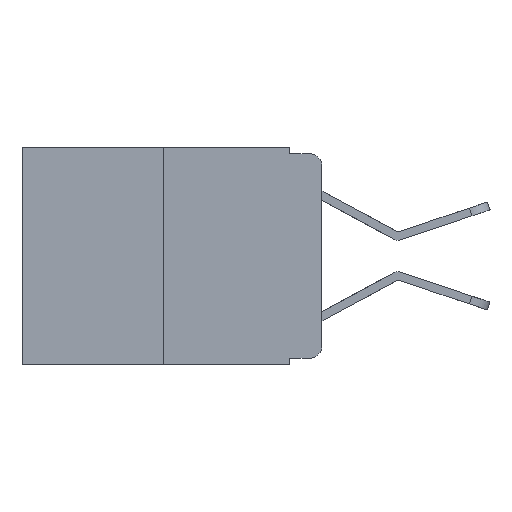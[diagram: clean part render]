
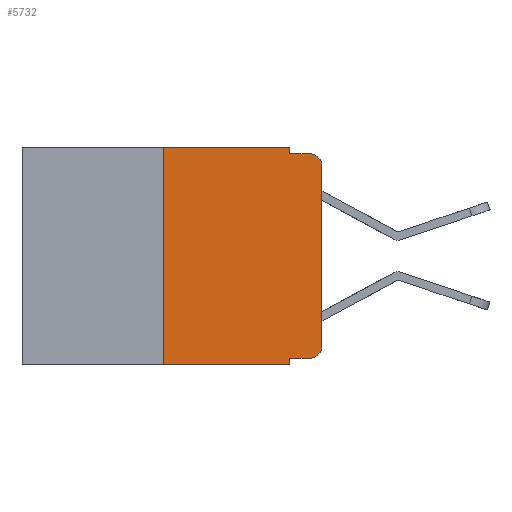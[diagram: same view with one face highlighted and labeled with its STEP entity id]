
A CAD part, left-side view. The second image highlights one B-rep face of the part: STEP entity #5732.
In plain terms, the highlighted planar face has unit normal (-1, 0, 0).
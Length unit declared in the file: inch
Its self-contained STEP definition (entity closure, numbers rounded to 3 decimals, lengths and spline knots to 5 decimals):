
#73 = LINE ( 'NONE', #10093, #9554 ) ;
#225 = VERTEX_POINT ( 'NONE', #10818 ) ;
#378 = EDGE_CURVE ( 'NONE', #3443, #225, #941, .T. ) ;
#417 = VECTOR ( 'NONE', #4463, 39.37008 ) ;
#472 = ORIENTED_EDGE ( 'NONE', *, *, #11811, .T. ) ;
#626 = VECTOR ( 'NONE', #1200, 39.37008 ) ;
#719 = CARTESIAN_POINT ( 'NONE',  ( 0., 0.051, -0.01 ) ) ;
#941 = LINE ( 'NONE', #6749, #626 ) ;
#1099 = VECTOR ( 'NONE', #4678, 39.37008 ) ;
#1198 = ORIENTED_EDGE ( 'NONE', *, *, #8436, .F. ) ;
#1200 = DIRECTION ( 'NONE',  ( 0., -1., 0. ) ) ;
#1203 = LINE ( 'NONE', #6163, #10564 ) ;
#1579 = VERTEX_POINT ( 'NONE', #11985 ) ;
#1754 = LINE ( 'NONE', #3778, #6861 ) ;
#1831 = AXIS2_PLACEMENT_3D ( 'NONE', #8529, #10321, #4838 ) ;
#1996 = VECTOR ( 'NONE', #5301, 39.37008 ) ;
#2070 = VERTEX_POINT ( 'NONE', #5599 ) ;
#2084 = EDGE_CURVE ( 'NONE', #9857, #3443, #4594, .T. ) ;
#2336 = AXIS2_PLACEMENT_3D ( 'NONE', #2449, #9038, #3432 ) ;
#2449 = CARTESIAN_POINT ( 'NONE',  ( 0., 0.02, -0.313 ) ) ;
#2727 = CARTESIAN_POINT ( 'NONE',  ( 0., 0.051, -0.01 ) ) ;
#2762 = ORIENTED_EDGE ( 'NONE', *, *, #378, .F. ) ;
#2826 = ORIENTED_EDGE ( 'NONE', *, *, #7855, .T. ) ;
#2958 = ORIENTED_EDGE ( 'NONE', *, *, #2084, .F. ) ;
#3263 = VERTEX_POINT ( 'NONE', #11679 ) ;
#3432 = DIRECTION ( 'NONE',  ( 0., 0., -1. ) ) ;
#3443 = VERTEX_POINT ( 'NONE', #3792 ) ;
#3673 = VERTEX_POINT ( 'NONE', #11362 ) ;
#3778 = CARTESIAN_POINT ( 'NONE',  ( 0., 0.473, -0.343 ) ) ;
#3792 = CARTESIAN_POINT ( 'NONE',  ( 0., 0.25, 0. ) ) ;
#3833 = EDGE_CURVE ( 'NONE', #1579, #6794, #1203, .T. ) ;
#3937 = LINE ( 'NONE', #7773, #8598 ) ;
#4463 = DIRECTION ( 'NONE',  ( 0., 0., -1. ) ) ;
#4594 = LINE ( 'NONE', #5342, #1996 ) ;
#4678 = DIRECTION ( 'NONE',  ( 0., -1., 0. ) ) ;
#4739 = DIRECTION ( 'NONE',  ( 0., -1., 0. ) ) ;
#4838 = DIRECTION ( 'NONE',  ( 0., 0., -1. ) ) ;
#5301 = DIRECTION ( 'NONE',  ( 0., 0., 1. ) ) ;
#5342 = CARTESIAN_POINT ( 'NONE',  ( 0., 0.25, 0. ) ) ;
#5568 = EDGE_CURVE ( 'NONE', #2070, #3673, #73, .T. ) ;
#5577 = CARTESIAN_POINT ( 'NONE',  ( 0., 0.02, -0.03 ) ) ;
#5599 = CARTESIAN_POINT ( 'NONE',  ( 0., 0., -0.313 ) ) ;
#5692 = FACE_OUTER_BOUND ( 'NONE', #7535, .T. ) ;
#5732 = ADVANCED_FACE ( 'NONE', ( #5692 ), #7590, .F. ) ;
#5830 = ORIENTED_EDGE ( 'NONE', *, *, #10685, .T. ) ;
#6163 = CARTESIAN_POINT ( 'NONE',  ( 0., 0.051, -0.333 ) ) ;
#6523 = ORIENTED_EDGE ( 'NONE', *, *, #7407, .F. ) ;
#6531 = DIRECTION ( 'NONE',  ( 0., 0., -1. ) ) ;
#6563 = VERTEX_POINT ( 'NONE', #7012 ) ;
#6716 = AXIS2_PLACEMENT_3D ( 'NONE', #5577, #11857, #6531 ) ;
#6749 = CARTESIAN_POINT ( 'NONE',  ( 0., 0.473, 0. ) ) ;
#6794 = VERTEX_POINT ( 'NONE', #7331 ) ;
#6861 = VECTOR ( 'NONE', #4739, 39.37008 ) ;
#7012 = CARTESIAN_POINT ( 'NONE',  ( 0., 0.051, -0.343 ) ) ;
#7082 = CIRCLE ( 'NONE', #2336, 0.02 ) ;
#7331 = CARTESIAN_POINT ( 'NONE',  ( 0., 0.02, -0.333 ) ) ;
#7407 = EDGE_CURVE ( 'NONE', #11214, #3263, #8666, .T. ) ;
#7535 = EDGE_LOOP ( 'NONE', ( #8572, #472, #6523, #8661, #2762, #2958, #5830, #1198, #8454, #2826 ) ) ;
#7590 = PLANE ( 'NONE',  #1831 ) ;
#7773 = CARTESIAN_POINT ( 'NONE',  ( 0., 0.051, 0. ) ) ;
#7855 = EDGE_CURVE ( 'NONE', #6794, #2070, #7082, .T. ) ;
#8058 = LINE ( 'NONE', #9969, #417 ) ;
#8436 = EDGE_CURVE ( 'NONE', #1579, #6563, #8058, .T. ) ;
#8454 = ORIENTED_EDGE ( 'NONE', *, *, #3833, .T. ) ;
#8529 = CARTESIAN_POINT ( 'NONE',  ( 0., 0.473, 0. ) ) ;
#8572 = ORIENTED_EDGE ( 'NONE', *, *, #5568, .T. ) ;
#8598 = VECTOR ( 'NONE', #8677, 39.37008 ) ;
#8661 = ORIENTED_EDGE ( 'NONE', *, *, #8752, .F. ) ;
#8666 = LINE ( 'NONE', #2727, #1099 ) ;
#8677 = DIRECTION ( 'NONE',  ( 0., 0., -1. ) ) ;
#8752 = EDGE_CURVE ( 'NONE', #225, #11214, #3937, .T. ) ;
#9038 = DIRECTION ( 'NONE',  ( -1., 0., 0. ) ) ;
#9554 = VECTOR ( 'NONE', #10971, 39.37008 ) ;
#9857 = VERTEX_POINT ( 'NONE', #11450 ) ;
#9969 = CARTESIAN_POINT ( 'NONE',  ( 0., 0.051, 0. ) ) ;
#10093 = CARTESIAN_POINT ( 'NONE',  ( 0., 0., 0. ) ) ;
#10321 = DIRECTION ( 'NONE',  ( 1., 0., 0. ) ) ;
#10500 = CIRCLE ( 'NONE', #6716, 0.02 ) ;
#10564 = VECTOR ( 'NONE', #11556, 39.37008 ) ;
#10685 = EDGE_CURVE ( 'NONE', #9857, #6563, #1754, .T. ) ;
#10818 = CARTESIAN_POINT ( 'NONE',  ( 0., 0.051, 0. ) ) ;
#10971 = DIRECTION ( 'NONE',  ( 0., 0., 1. ) ) ;
#11214 = VERTEX_POINT ( 'NONE', #719 ) ;
#11362 = CARTESIAN_POINT ( 'NONE',  ( 0., 0., -0.03 ) ) ;
#11450 = CARTESIAN_POINT ( 'NONE',  ( 0., 0.25, -0.343 ) ) ;
#11556 = DIRECTION ( 'NONE',  ( 0., -1., 0. ) ) ;
#11679 = CARTESIAN_POINT ( 'NONE',  ( 0., 0.02, -0.01 ) ) ;
#11811 = EDGE_CURVE ( 'NONE', #3673, #3263, #10500, .T. ) ;
#11857 = DIRECTION ( 'NONE',  ( -1., 0., 0. ) ) ;
#11985 = CARTESIAN_POINT ( 'NONE',  ( 0., 0.051, -0.333 ) ) ;
